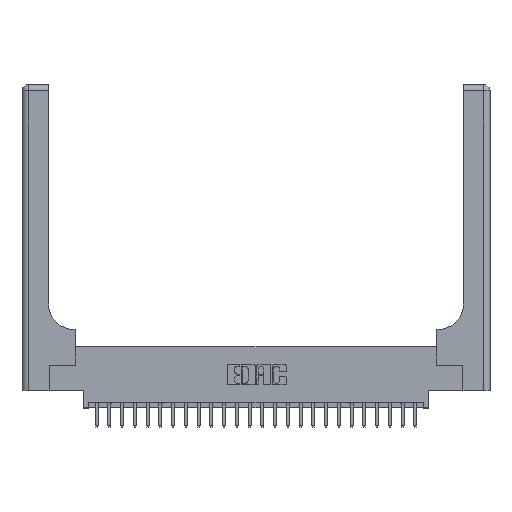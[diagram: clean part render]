
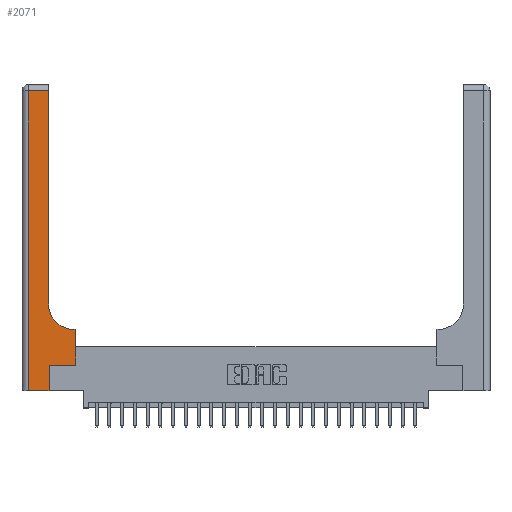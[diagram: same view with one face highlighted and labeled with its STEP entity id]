
A CAD part, top view. The second image highlights one B-rep face of the part: STEP entity #2071.
In plain terms, the highlighted planar face has unit normal (0, 0, 1).
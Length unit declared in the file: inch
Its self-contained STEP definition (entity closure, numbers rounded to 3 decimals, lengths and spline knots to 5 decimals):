
#988 = DIRECTION ( 'NONE',  ( 1., 0., 0. ) ) ;
#1095 = VECTOR ( 'NONE', #19142, 39.37008 ) ;
#1550 = CIRCLE ( 'NONE', #14052, 0.25 ) ;
#2071 = ADVANCED_FACE ( 'NONE', ( #22291 ), #10392, .F. ) ;
#2904 = CARTESIAN_POINT ( 'NONE',  ( 0.26, 0.85, 0.37 ) ) ;
#3008 = DIRECTION ( 'NONE',  ( 0., 1., 0. ) ) ;
#3279 = ORIENTED_EDGE ( 'NONE', *, *, #24870, .T. ) ;
#3380 = AXIS2_PLACEMENT_3D ( 'NONE', #19898, #18209, #4965 ) ;
#3411 = CARTESIAN_POINT ( 'NONE',  ( 0.26, 2.94, 0.37 ) ) ;
#3721 = LINE ( 'NONE', #11415, #1095 ) ;
#4382 = CARTESIAN_POINT ( 'NONE',  ( 0.51, 0.6, 0.37 ) ) ;
#4518 = EDGE_LOOP ( 'NONE', ( #24121, #23168, #7906, #5426, #3279, #19059, #5261, #8422, #22919 ) ) ;
#4965 = DIRECTION ( 'NONE',  ( -1., 0., 0. ) ) ;
#5047 = CARTESIAN_POINT ( 'NONE',  ( 0.265, 0., 0.37 ) ) ;
#5261 = ORIENTED_EDGE ( 'NONE', *, *, #20111, .T. ) ;
#5426 = ORIENTED_EDGE ( 'NONE', *, *, #6549, .T. ) ;
#5737 = CARTESIAN_POINT ( 'NONE',  ( 0.51, 0.85, 0.37 ) ) ;
#6167 = CARTESIAN_POINT ( 'NONE',  ( 0.528, 0.25, 0.37 ) ) ;
#6549 = EDGE_CURVE ( 'NONE', #20944, #7127, #15410, .T. ) ;
#6577 = CARTESIAN_POINT ( 'NONE',  ( 0.265, 0.25, 0.37 ) ) ;
#7127 = VERTEX_POINT ( 'NONE', #13935 ) ;
#7745 = VECTOR ( 'NONE', #988, 39.37008 ) ;
#7906 = ORIENTED_EDGE ( 'NONE', *, *, #18484, .T. ) ;
#7994 = DIRECTION ( 'NONE',  ( 0., -1., 0. ) ) ;
#8422 = ORIENTED_EDGE ( 'NONE', *, *, #18351, .T. ) ;
#8570 = VECTOR ( 'NONE', #3008, 39.37008 ) ;
#8818 = LINE ( 'NONE', #5047, #8570 ) ;
#9708 = VECTOR ( 'NONE', #10735, 39.37008 ) ;
#10316 = VERTEX_POINT ( 'NONE', #6167 ) ;
#10392 = PLANE ( 'NONE',  #3380 ) ;
#10735 = DIRECTION ( 'NONE',  ( 0., 1., 0. ) ) ;
#10790 = LINE ( 'NONE', #18239, #15713 ) ;
#11415 = CARTESIAN_POINT ( 'NONE',  ( 0.26, 0.6, 0.37 ) ) ;
#11644 = DIRECTION ( 'NONE',  ( 1., 0., 0. ) ) ;
#11662 = CARTESIAN_POINT ( 'NONE',  ( 0.528, 0.25, 0.37 ) ) ;
#11961 = EDGE_CURVE ( 'NONE', #19122, #19967, #10790, .T. ) ;
#12897 = VERTEX_POINT ( 'NONE', #2904 ) ;
#13009 = LINE ( 'NONE', #18704, #9708 ) ;
#13240 = CARTESIAN_POINT ( 'NONE',  ( 0., 0., 0.37 ) ) ;
#13700 = VECTOR ( 'NONE', #19019, 39.37008 ) ;
#13935 = CARTESIAN_POINT ( 'NONE',  ( 0.265, 0., 0.37 ) ) ;
#14052 = AXIS2_PLACEMENT_3D ( 'NONE', #5737, #21157, #11644 ) ;
#14314 = VECTOR ( 'NONE', #20844, 39.37008 ) ;
#14467 = CARTESIAN_POINT ( 'NONE',  ( 0.06, 0., 0.37 ) ) ;
#15363 = CARTESIAN_POINT ( 'NONE',  ( 0.265, 0.25, 0.37 ) ) ;
#15410 = LINE ( 'NONE', #13240, #14314 ) ;
#15713 = VECTOR ( 'NONE', #16732, 39.37008 ) ;
#15825 = LINE ( 'NONE', #17579, #17266 ) ;
#16210 = VERTEX_POINT ( 'NONE', #4382 ) ;
#16513 = VERTEX_POINT ( 'NONE', #15363 ) ;
#16732 = DIRECTION ( 'NONE',  ( -1., 0., 0. ) ) ;
#17207 = EDGE_CURVE ( 'NONE', #16210, #12897, #1550, .T. ) ;
#17266 = VECTOR ( 'NONE', #7994, 39.37008 ) ;
#17579 = CARTESIAN_POINT ( 'NONE',  ( 0.06, 3., 0.37 ) ) ;
#18209 = DIRECTION ( 'NONE',  ( 0., 0., -1. ) ) ;
#18239 = CARTESIAN_POINT ( 'NONE',  ( 0., 2.94, 0.37 ) ) ;
#18351 = EDGE_CURVE ( 'NONE', #21083, #16210, #3721, .T. ) ;
#18372 = CARTESIAN_POINT ( 'NONE',  ( 0.528, 0.6, 0.37 ) ) ;
#18484 = EDGE_CURVE ( 'NONE', #19967, #20944, #15825, .T. ) ;
#18704 = CARTESIAN_POINT ( 'NONE',  ( 0.26, 3., 0.37 ) ) ;
#19019 = DIRECTION ( 'NONE',  ( 0., 1., 0. ) ) ;
#19059 = ORIENTED_EDGE ( 'NONE', *, *, #24202, .T. ) ;
#19122 = VERTEX_POINT ( 'NONE', #3411 ) ;
#19142 = DIRECTION ( 'NONE',  ( -1., 0., 0. ) ) ;
#19277 = LINE ( 'NONE', #11662, #13700 ) ;
#19898 = CARTESIAN_POINT ( 'NONE',  ( 0., 3., 0.37 ) ) ;
#19967 = VERTEX_POINT ( 'NONE', #20530 ) ;
#20111 = EDGE_CURVE ( 'NONE', #10316, #21083, #19277, .T. ) ;
#20530 = CARTESIAN_POINT ( 'NONE',  ( 0.06, 2.94, 0.37 ) ) ;
#20844 = DIRECTION ( 'NONE',  ( 1., 0., 0. ) ) ;
#20944 = VERTEX_POINT ( 'NONE', #14467 ) ;
#21083 = VERTEX_POINT ( 'NONE', #18372 ) ;
#21157 = DIRECTION ( 'NONE',  ( 0., 0., -1. ) ) ;
#22017 = LINE ( 'NONE', #6577, #7745 ) ;
#22291 = FACE_OUTER_BOUND ( 'NONE', #4518, .T. ) ;
#22919 = ORIENTED_EDGE ( 'NONE', *, *, #17207, .T. ) ;
#23168 = ORIENTED_EDGE ( 'NONE', *, *, #11961, .T. ) ;
#23327 = EDGE_CURVE ( 'NONE', #12897, #19122, #13009, .T. ) ;
#24121 = ORIENTED_EDGE ( 'NONE', *, *, #23327, .T. ) ;
#24202 = EDGE_CURVE ( 'NONE', #16513, #10316, #22017, .T. ) ;
#24870 = EDGE_CURVE ( 'NONE', #7127, #16513, #8818, .T. ) ;
